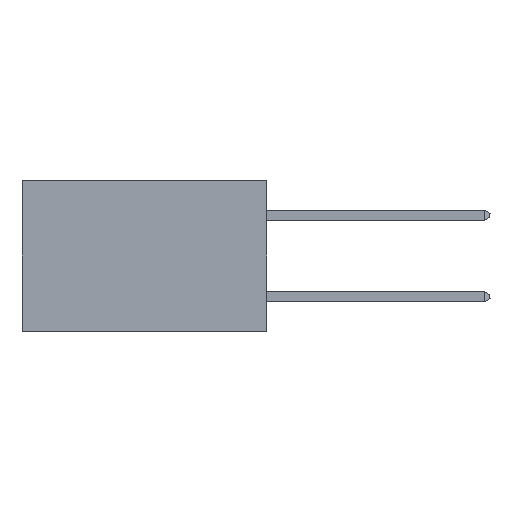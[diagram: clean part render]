
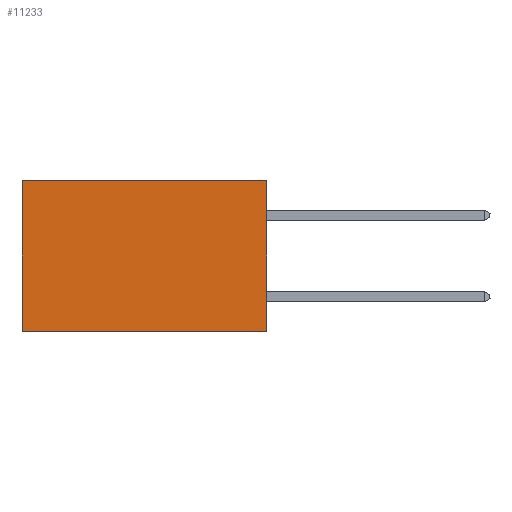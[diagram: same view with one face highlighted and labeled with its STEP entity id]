
A CAD part, left-side view. The second image highlights one B-rep face of the part: STEP entity #11233.
In plain terms, the highlighted planar face has unit normal (-1, 0, 0).
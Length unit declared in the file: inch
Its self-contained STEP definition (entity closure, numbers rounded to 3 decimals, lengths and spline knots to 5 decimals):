
#1305 = DIRECTION ( 'NONE',  ( 0., 1., 0. ) ) ;
#1435 = CARTESIAN_POINT ( 'NONE',  ( 0.2875, 0., 0. ) ) ;
#2455 = CARTESIAN_POINT ( 'NONE',  ( 0.2875, 0.6, 0. ) ) ;
#2786 = VERTEX_POINT ( 'NONE', #21217 ) ;
#3551 = AXIS2_PLACEMENT_3D ( 'NONE', #1435, #12707, #20268 ) ;
#3645 = CARTESIAN_POINT ( 'NONE',  ( 0.2875, 0.6, -0.37 ) ) ;
#4526 = LINE ( 'NONE', #7354, #6564 ) ;
#4797 = DIRECTION ( 'NONE',  ( 0., 1., 0. ) ) ;
#6564 = VECTOR ( 'NONE', #20468, 39.37008 ) ;
#7354 = CARTESIAN_POINT ( 'NONE',  ( 0.2875, 0., 0. ) ) ;
#7749 = CARTESIAN_POINT ( 'NONE',  ( 0.2875, 0., 0. ) ) ;
#9102 = VECTOR ( 'NONE', #4797, 39.37008 ) ;
#9205 = EDGE_LOOP ( 'NONE', ( #12958, #11764, #10300, #13269 ) ) ;
#10300 = ORIENTED_EDGE ( 'NONE', *, *, #13148, .F. ) ;
#10478 = CARTESIAN_POINT ( 'NONE',  ( 0.2875, 0.6, 0. ) ) ;
#11026 = EDGE_CURVE ( 'NONE', #23987, #20317, #12761, .T. ) ;
#11221 = CARTESIAN_POINT ( 'NONE',  ( 0.2875, 0., 0. ) ) ;
#11233 = ADVANCED_FACE ( 'NONE', ( #17439 ), #18295, .F. ) ;
#11764 = ORIENTED_EDGE ( 'NONE', *, *, #21092, .F. ) ;
#12163 = VECTOR ( 'NONE', #1305, 39.37008 ) ;
#12506 = VECTOR ( 'NONE', #21872, 39.37008 ) ;
#12707 = DIRECTION ( 'NONE',  ( 1., 0., 0. ) ) ;
#12761 = LINE ( 'NONE', #7749, #12163 ) ;
#12888 = LINE ( 'NONE', #19620, #9102 ) ;
#12958 = ORIENTED_EDGE ( 'NONE', *, *, #22387, .T. ) ;
#13148 = EDGE_CURVE ( 'NONE', #23987, #2786, #4526, .T. ) ;
#13269 = ORIENTED_EDGE ( 'NONE', *, *, #11026, .T. ) ;
#17439 = FACE_OUTER_BOUND ( 'NONE', #9205, .T. ) ;
#18295 = PLANE ( 'NONE',  #3551 ) ;
#19290 = VERTEX_POINT ( 'NONE', #3645 ) ;
#19620 = CARTESIAN_POINT ( 'NONE',  ( 0.2875, 0., -0.37 ) ) ;
#20268 = DIRECTION ( 'NONE',  ( 0., 0., -1. ) ) ;
#20317 = VERTEX_POINT ( 'NONE', #2455 ) ;
#20468 = DIRECTION ( 'NONE',  ( 0., 0., -1. ) ) ;
#21092 = EDGE_CURVE ( 'NONE', #2786, #19290, #12888, .T. ) ;
#21217 = CARTESIAN_POINT ( 'NONE',  ( 0.2875, 0., -0.37 ) ) ;
#21872 = DIRECTION ( 'NONE',  ( 0., 0., -1. ) ) ;
#22387 = EDGE_CURVE ( 'NONE', #20317, #19290, #23997, .T. ) ;
#23987 = VERTEX_POINT ( 'NONE', #11221 ) ;
#23997 = LINE ( 'NONE', #10478, #12506 ) ;
